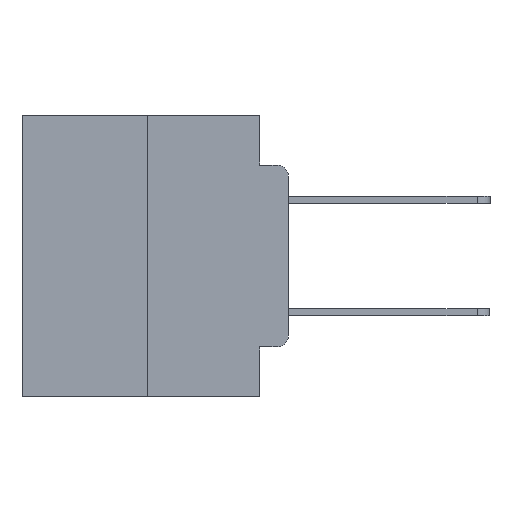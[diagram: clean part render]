
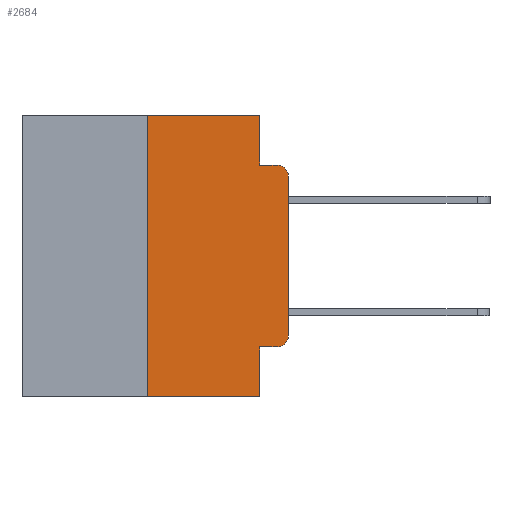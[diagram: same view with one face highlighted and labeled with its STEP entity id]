
A CAD part, left-side view. The second image highlights one B-rep face of the part: STEP entity #2684.
In plain terms, the highlighted planar face has unit normal (-1, 0, 0).
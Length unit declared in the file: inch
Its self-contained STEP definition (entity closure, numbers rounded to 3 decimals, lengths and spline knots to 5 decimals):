
#520 = ORIENTED_EDGE ( 'NONE', *, *, #8050, .T. ) ;
#668 = CARTESIAN_POINT ( 'NONE',  ( 0., 0.02, -0.0885 ) ) ;
#669 = VECTOR ( 'NONE', #14015, 39.37008 ) ;
#683 = EDGE_LOOP ( 'NONE', ( #520, #5193, #14001, #5392, #14798, #12552, #5151, #10064, #11400, #13987 ) ) ;
#765 = DIRECTION ( 'NONE',  ( 0., 0., 1. ) ) ;
#1788 = DIRECTION ( 'NONE',  ( 0., 0., -1. ) ) ;
#1807 = LINE ( 'NONE', #17149, #11950 ) ;
#1968 = CARTESIAN_POINT ( 'NONE',  ( 0., 0.051, 0. ) ) ;
#2271 = DIRECTION ( 'NONE',  ( 0., -1., 0. ) ) ;
#2607 = DIRECTION ( 'NONE',  ( 0., -1., 0. ) ) ;
#2680 = DIRECTION ( 'NONE',  ( 0., 0., -1. ) ) ;
#2684 = ADVANCED_FACE ( 'NONE', ( #26329 ), #15384, .F. ) ;
#3214 = CARTESIAN_POINT ( 'NONE',  ( 0., 0.051, -0.0885 ) ) ;
#3323 = CARTESIAN_POINT ( 'NONE',  ( 0., 0., -0.3915 ) ) ;
#3680 = DIRECTION ( 'NONE',  ( -1., 0., 0. ) ) ;
#3949 = CARTESIAN_POINT ( 'NONE',  ( 0., 0.473, 0. ) ) ;
#4189 = EDGE_CURVE ( 'NONE', #24258, #14993, #23444, .T. ) ;
#4560 = VERTEX_POINT ( 'NONE', #18021 ) ;
#5075 = AXIS2_PLACEMENT_3D ( 'NONE', #27040, #14621, #1788 ) ;
#5151 = ORIENTED_EDGE ( 'NONE', *, *, #18510, .T. ) ;
#5193 = ORIENTED_EDGE ( 'NONE', *, *, #25334, .T. ) ;
#5240 = LINE ( 'NONE', #5592, #20002 ) ;
#5392 = ORIENTED_EDGE ( 'NONE', *, *, #16964, .F. ) ;
#5592 = CARTESIAN_POINT ( 'NONE',  ( 0., 0.051, 0. ) ) ;
#5600 = LINE ( 'NONE', #19599, #27213 ) ;
#7162 = EDGE_CURVE ( 'NONE', #8886, #24258, #26831, .T. ) ;
#7585 = LINE ( 'NONE', #3949, #13200 ) ;
#7734 = DIRECTION ( 'NONE',  ( 0., -1., 0. ) ) ;
#8035 = VERTEX_POINT ( 'NONE', #668 ) ;
#8050 = EDGE_CURVE ( 'NONE', #14993, #17481, #26779, .T. ) ;
#8282 = LINE ( 'NONE', #17469, #22952 ) ;
#8886 = VERTEX_POINT ( 'NONE', #16153 ) ;
#9220 = DIRECTION ( 'NONE',  ( 0., 0., 1. ) ) ;
#10017 = EDGE_CURVE ( 'NONE', #8886, #15448, #17044, .T. ) ;
#10064 = ORIENTED_EDGE ( 'NONE', *, *, #10017, .F. ) ;
#10067 = CARTESIAN_POINT ( 'NONE',  ( 0., 0.25, -0.5 ) ) ;
#10194 = AXIS2_PLACEMENT_3D ( 'NONE', #16404, #3680, #18441 ) ;
#11341 = CARTESIAN_POINT ( 'NONE',  ( 0., 0.473, 0. ) ) ;
#11400 = ORIENTED_EDGE ( 'NONE', *, *, #7162, .T. ) ;
#11950 = VECTOR ( 'NONE', #2271, 39.37008 ) ;
#12552 = ORIENTED_EDGE ( 'NONE', *, *, #14196, .F. ) ;
#13200 = VECTOR ( 'NONE', #27004, 39.37008 ) ;
#13656 = CARTESIAN_POINT ( 'NONE',  ( 0., 0., 0. ) ) ;
#13748 = VERTEX_POINT ( 'NONE', #10067 ) ;
#13943 = VERTEX_POINT ( 'NONE', #1968 ) ;
#13987 = ORIENTED_EDGE ( 'NONE', *, *, #4189, .T. ) ;
#14001 = ORIENTED_EDGE ( 'NONE', *, *, #22549, .F. ) ;
#14015 = DIRECTION ( 'NONE',  ( 0., 0., -1. ) ) ;
#14113 = CARTESIAN_POINT ( 'NONE',  ( 0., 0.051, 0. ) ) ;
#14196 = EDGE_CURVE ( 'NONE', #13748, #4560, #5600, .T. ) ;
#14621 = DIRECTION ( 'NONE',  ( -1., 0., 0. ) ) ;
#14798 = ORIENTED_EDGE ( 'NONE', *, *, #18915, .F. ) ;
#14993 = VERTEX_POINT ( 'NONE', #3323 ) ;
#15211 = CARTESIAN_POINT ( 'NONE',  ( 0., 0.02, -0.4115 ) ) ;
#15384 = PLANE ( 'NONE',  #23899 ) ;
#15448 = VERTEX_POINT ( 'NONE', #23780 ) ;
#15471 = DIRECTION ( 'NONE',  ( 1., 0., 0. ) ) ;
#16153 = CARTESIAN_POINT ( 'NONE',  ( 0., 0.051, -0.4115 ) ) ;
#16404 = CARTESIAN_POINT ( 'NONE',  ( 0., 0.02, -0.3915 ) ) ;
#16964 = EDGE_CURVE ( 'NONE', #13943, #25120, #5240, .T. ) ;
#17044 = LINE ( 'NONE', #14113, #669 ) ;
#17149 = CARTESIAN_POINT ( 'NONE',  ( 0., 0.051, -0.0885 ) ) ;
#17469 = CARTESIAN_POINT ( 'NONE',  ( 0., 0.473, -0.5 ) ) ;
#17481 = VERTEX_POINT ( 'NONE', #20031 ) ;
#18021 = CARTESIAN_POINT ( 'NONE',  ( 0., 0.25, 0. ) ) ;
#18441 = DIRECTION ( 'NONE',  ( 0., 0., -1. ) ) ;
#18510 = EDGE_CURVE ( 'NONE', #13748, #15448, #8282, .T. ) ;
#18915 = EDGE_CURVE ( 'NONE', #4560, #13943, #7585, .T. ) ;
#19599 = CARTESIAN_POINT ( 'NONE',  ( 0., 0.25, 0. ) ) ;
#20002 = VECTOR ( 'NONE', #20158, 39.37008 ) ;
#20031 = CARTESIAN_POINT ( 'NONE',  ( 0., 0., -0.1085 ) ) ;
#20158 = DIRECTION ( 'NONE',  ( 0., 0., -1. ) ) ;
#20184 = CARTESIAN_POINT ( 'NONE',  ( 0., 0.051, -0.4115 ) ) ;
#20582 = VECTOR ( 'NONE', #765, 39.37008 ) ;
#22549 = EDGE_CURVE ( 'NONE', #25120, #8035, #1807, .T. ) ;
#22952 = VECTOR ( 'NONE', #2607, 39.37008 ) ;
#23444 = CIRCLE ( 'NONE', #10194, 0.02 ) ;
#23780 = CARTESIAN_POINT ( 'NONE',  ( 0., 0.051, -0.5 ) ) ;
#23899 = AXIS2_PLACEMENT_3D ( 'NONE', #11341, #15471, #2680 ) ;
#24258 = VERTEX_POINT ( 'NONE', #15211 ) ;
#25120 = VERTEX_POINT ( 'NONE', #3214 ) ;
#25334 = EDGE_CURVE ( 'NONE', #17481, #8035, #25460, .T. ) ;
#25460 = CIRCLE ( 'NONE', #5075, 0.02 ) ;
#26155 = VECTOR ( 'NONE', #7734, 39.37008 ) ;
#26329 = FACE_OUTER_BOUND ( 'NONE', #683, .T. ) ;
#26779 = LINE ( 'NONE', #13656, #20582 ) ;
#26831 = LINE ( 'NONE', #20184, #26155 ) ;
#27004 = DIRECTION ( 'NONE',  ( 0., -1., 0. ) ) ;
#27040 = CARTESIAN_POINT ( 'NONE',  ( 0., 0.02, -0.1085 ) ) ;
#27213 = VECTOR ( 'NONE', #9220, 39.37008 ) ;
